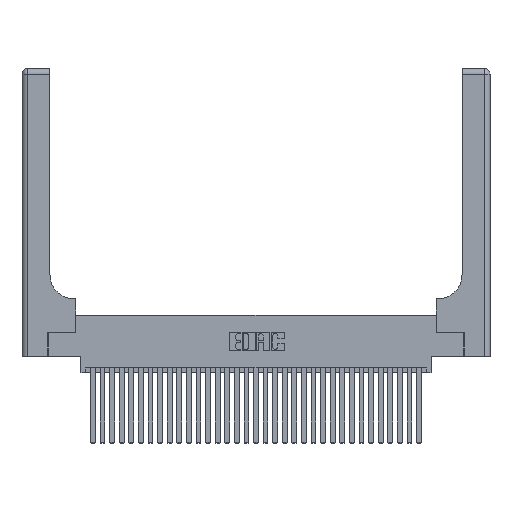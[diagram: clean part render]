
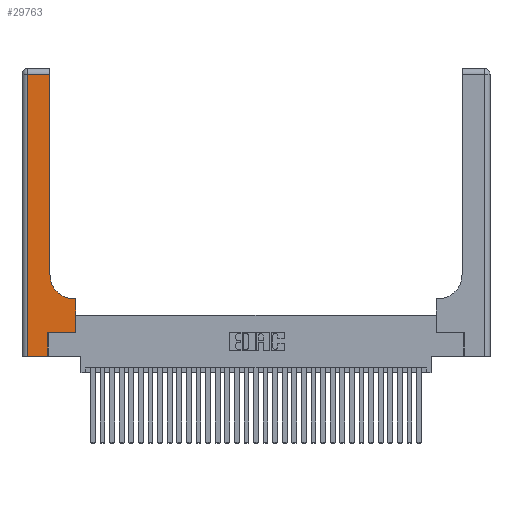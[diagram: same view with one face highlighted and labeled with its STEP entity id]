
A CAD part, top view. The second image highlights one B-rep face of the part: STEP entity #29763.
In plain terms, the highlighted planar face has unit normal (0, 0, 1).
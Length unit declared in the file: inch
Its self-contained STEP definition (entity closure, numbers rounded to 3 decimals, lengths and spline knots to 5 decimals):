
#360 = DIRECTION ( 'NONE',  ( 0., 1., 0. ) ) ;
#614 = CARTESIAN_POINT ( 'NONE',  ( 0.269, 0., 0.37 ) ) ;
#1634 = VERTEX_POINT ( 'NONE', #30719 ) ;
#1696 = LINE ( 'NONE', #14362, #7803 ) ;
#2264 = CARTESIAN_POINT ( 'NONE',  ( 0., 3., 0.37 ) ) ;
#2597 = AXIS2_PLACEMENT_3D ( 'NONE', #2264, #2699, #31131 ) ;
#2699 = DIRECTION ( 'NONE',  ( 0., 0., -1. ) ) ;
#2756 = LINE ( 'NONE', #6816, #14962 ) ;
#3568 = ORIENTED_EDGE ( 'NONE', *, *, #23403, .T. ) ;
#3626 = CARTESIAN_POINT ( 'NONE',  ( 0., 2.94, 0.37 ) ) ;
#3739 = CARTESIAN_POINT ( 'NONE',  ( 0.5415, 0.6, 0.37 ) ) ;
#4987 = ORIENTED_EDGE ( 'NONE', *, *, #12197, .T. ) ;
#5292 = LINE ( 'NONE', #26707, #30023 ) ;
#6174 = DIRECTION ( 'NONE',  ( -1., 0., 0. ) ) ;
#6816 = CARTESIAN_POINT ( 'NONE',  ( 0.269, 0., 0.37 ) ) ;
#7463 = VECTOR ( 'NONE', #27000, 39.37008 ) ;
#7507 = CARTESIAN_POINT ( 'NONE',  ( 0.5585, 0.25, 0.37 ) ) ;
#7673 = AXIS2_PLACEMENT_3D ( 'NONE', #10931, #31619, #31953 ) ;
#7746 = ORIENTED_EDGE ( 'NONE', *, *, #9306, .T. ) ;
#7803 = VECTOR ( 'NONE', #16497, 39.37008 ) ;
#8539 = DIRECTION ( 'NONE',  ( 0., 1., 0. ) ) ;
#9295 = ORIENTED_EDGE ( 'NONE', *, *, #28029, .T. ) ;
#9306 = EDGE_CURVE ( 'NONE', #26094, #28578, #25237, .T. ) ;
#10202 = CARTESIAN_POINT ( 'NONE',  ( 0.06, 3., 0.37 ) ) ;
#10931 = CARTESIAN_POINT ( 'NONE',  ( 0.5415, 0.85, 0.37 ) ) ;
#11061 = VERTEX_POINT ( 'NONE', #7507 ) ;
#12197 = EDGE_CURVE ( 'NONE', #28578, #30827, #2756, .T. ) ;
#12695 = ORIENTED_EDGE ( 'NONE', *, *, #19733, .T. ) ;
#12819 = PLANE ( 'NONE',  #2597 ) ;
#13719 = VECTOR ( 'NONE', #18972, 39.37008 ) ;
#14362 = CARTESIAN_POINT ( 'NONE',  ( 0.2915, 0.6, 0.37 ) ) ;
#14585 = CARTESIAN_POINT ( 'NONE',  ( 0.269, 0.25, 0.37 ) ) ;
#14589 = EDGE_CURVE ( 'NONE', #11061, #18467, #26119, .T. ) ;
#14672 = CARTESIAN_POINT ( 'NONE',  ( 0.5585, 0.6, 0.37 ) ) ;
#14962 = VECTOR ( 'NONE', #8539, 39.37008 ) ;
#16497 = DIRECTION ( 'NONE',  ( -1., 0., 0. ) ) ;
#16770 = DIRECTION ( 'NONE',  ( 0., 1., 0. ) ) ;
#16786 = CIRCLE ( 'NONE', #7673, 0.25 ) ;
#16840 = VECTOR ( 'NONE', #360, 39.37008 ) ;
#16842 = EDGE_LOOP ( 'NONE', ( #9295, #21691, #3568, #7746, #4987, #28225, #31975, #12695, #19714 ) ) ;
#18149 = EDGE_CURVE ( 'NONE', #24776, #1634, #16786, .T. ) ;
#18201 = EDGE_CURVE ( 'NONE', #29153, #33194, #20389, .T. ) ;
#18467 = VERTEX_POINT ( 'NONE', #14672 ) ;
#18972 = DIRECTION ( 'NONE',  ( 0., -1., 0. ) ) ;
#19714 = ORIENTED_EDGE ( 'NONE', *, *, #18149, .T. ) ;
#19733 = EDGE_CURVE ( 'NONE', #18467, #24776, #1696, .T. ) ;
#19774 = DIRECTION ( 'NONE',  ( 1., 0., 0. ) ) ;
#20389 = LINE ( 'NONE', #3626, #22837 ) ;
#21585 = VECTOR ( 'NONE', #19774, 39.37008 ) ;
#21691 = ORIENTED_EDGE ( 'NONE', *, *, #18201, .T. ) ;
#22837 = VECTOR ( 'NONE', #6174, 39.37008 ) ;
#22844 = FACE_OUTER_BOUND ( 'NONE', #16842, .T. ) ;
#23403 = EDGE_CURVE ( 'NONE', #33194, #26094, #25052, .T. ) ;
#24348 = CARTESIAN_POINT ( 'NONE',  ( 0.269, 0.25, 0.37 ) ) ;
#24776 = VERTEX_POINT ( 'NONE', #3739 ) ;
#25052 = LINE ( 'NONE', #10202, #13719 ) ;
#25237 = LINE ( 'NONE', #29346, #7463 ) ;
#25981 = CARTESIAN_POINT ( 'NONE',  ( 0.5585, 0.25, 0.37 ) ) ;
#26094 = VERTEX_POINT ( 'NONE', #26664 ) ;
#26119 = LINE ( 'NONE', #25981, #16840 ) ;
#26312 = EDGE_CURVE ( 'NONE', #30827, #11061, #29236, .T. ) ;
#26664 = CARTESIAN_POINT ( 'NONE',  ( 0.06, 0., 0.37 ) ) ;
#26707 = CARTESIAN_POINT ( 'NONE',  ( 0.2915, 3., 0.37 ) ) ;
#27000 = DIRECTION ( 'NONE',  ( 1., 0., 0. ) ) ;
#28029 = EDGE_CURVE ( 'NONE', #1634, #29153, #5292, .T. ) ;
#28225 = ORIENTED_EDGE ( 'NONE', *, *, #26312, .T. ) ;
#28578 = VERTEX_POINT ( 'NONE', #614 ) ;
#29153 = VERTEX_POINT ( 'NONE', #31393 ) ;
#29236 = LINE ( 'NONE', #14585, #21585 ) ;
#29346 = CARTESIAN_POINT ( 'NONE',  ( 0., 0., 0.37 ) ) ;
#29763 = ADVANCED_FACE ( 'NONE', ( #22844 ), #12819, .F. ) ;
#30023 = VECTOR ( 'NONE', #16770, 39.37008 ) ;
#30431 = CARTESIAN_POINT ( 'NONE',  ( 0.06, 2.94, 0.37 ) ) ;
#30719 = CARTESIAN_POINT ( 'NONE',  ( 0.2915, 0.85, 0.37 ) ) ;
#30827 = VERTEX_POINT ( 'NONE', #24348 ) ;
#31131 = DIRECTION ( 'NONE',  ( -1., 0., 0. ) ) ;
#31393 = CARTESIAN_POINT ( 'NONE',  ( 0.2915, 2.94, 0.37 ) ) ;
#31619 = DIRECTION ( 'NONE',  ( 0., 0., -1. ) ) ;
#31953 = DIRECTION ( 'NONE',  ( 1., 0., 0. ) ) ;
#31975 = ORIENTED_EDGE ( 'NONE', *, *, #14589, .T. ) ;
#33194 = VERTEX_POINT ( 'NONE', #30431 ) ;
